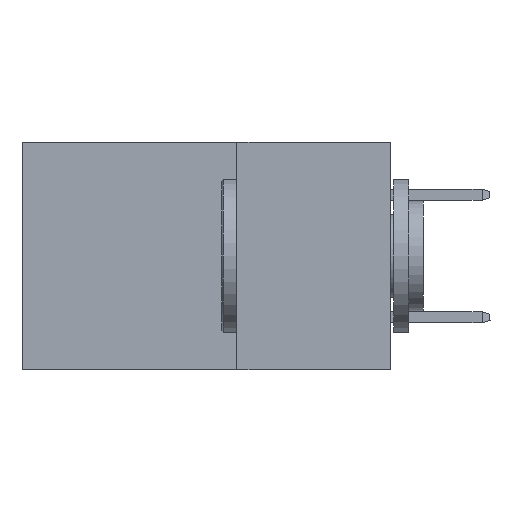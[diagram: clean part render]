
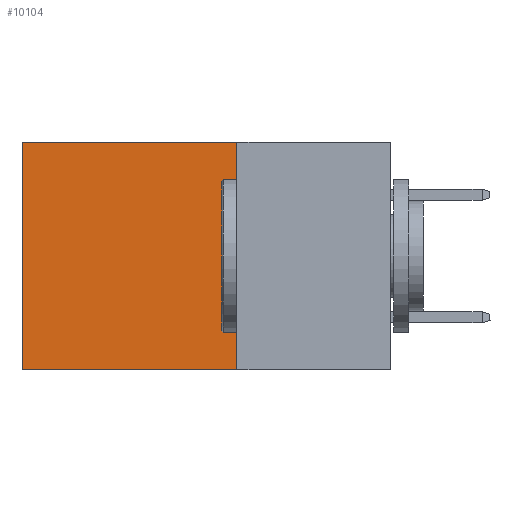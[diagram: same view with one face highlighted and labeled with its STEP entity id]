
A CAD part, left-side view. The second image highlights one B-rep face of the part: STEP entity #10104.
In plain terms, the highlighted planar face has unit normal (-1, 0, 0).
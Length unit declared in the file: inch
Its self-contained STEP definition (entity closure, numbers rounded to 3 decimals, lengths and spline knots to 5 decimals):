
#176 = LINE ( 'NONE', #5100, #5305 ) ;
#503 = AXIS2_PLACEMENT_3D ( 'NONE', #12562, #1805, #9003 ) ;
#543 = LINE ( 'NONE', #991, #11005 ) ;
#823 = LINE ( 'NONE', #1320, #3710 ) ;
#925 = DIRECTION ( 'NONE',  ( 0., 0., -1. ) ) ;
#991 = CARTESIAN_POINT ( 'NONE',  ( 0.2875, 0.25, 0. ) ) ;
#1142 = VERTEX_POINT ( 'NONE', #2001 ) ;
#1304 = DIRECTION ( 'NONE',  ( 0., 1., 0. ) ) ;
#1320 = CARTESIAN_POINT ( 'NONE',  ( 0.2875, 0.25, -0.37 ) ) ;
#1624 = LINE ( 'NONE', #2728, #6925 ) ;
#1805 = DIRECTION ( 'NONE',  ( 1., 0., 0. ) ) ;
#1990 = EDGE_CURVE ( 'NONE', #1142, #12833, #543, .T. ) ;
#2001 = CARTESIAN_POINT ( 'NONE',  ( 0.2875, 0.25, 0. ) ) ;
#2570 = ORIENTED_EDGE ( 'NONE', *, *, #1990, .F. ) ;
#2582 = EDGE_CURVE ( 'NONE', #1142, #4583, #176, .T. ) ;
#2728 = CARTESIAN_POINT ( 'NONE',  ( 0.2875, 0.6, 0. ) ) ;
#3677 = ORIENTED_EDGE ( 'NONE', *, *, #11192, .T. ) ;
#3710 = VECTOR ( 'NONE', #1304, 39.37008 ) ;
#3799 = DIRECTION ( 'NONE',  ( 0., 0., -1. ) ) ;
#4583 = VERTEX_POINT ( 'NONE', #12522 ) ;
#5075 = DIRECTION ( 'NONE',  ( 0., 1., 0. ) ) ;
#5100 = CARTESIAN_POINT ( 'NONE',  ( 0.2875, 0.25, 0. ) ) ;
#5305 = VECTOR ( 'NONE', #5075, 39.37008 ) ;
#5379 = CARTESIAN_POINT ( 'NONE',  ( 0.2875, 0.25, -0.37 ) ) ;
#6227 = EDGE_CURVE ( 'NONE', #12833, #11736, #823, .T. ) ;
#6925 = VECTOR ( 'NONE', #3799, 39.37008 ) ;
#7273 = FACE_OUTER_BOUND ( 'NONE', #10114, .T. ) ;
#8048 = PLANE ( 'NONE',  #503 ) ;
#9003 = DIRECTION ( 'NONE',  ( 0., 0., -1. ) ) ;
#9690 = CARTESIAN_POINT ( 'NONE',  ( 0.2875, 0.6, -0.37 ) ) ;
#10104 = ADVANCED_FACE ( 'NONE', ( #7273 ), #8048, .F. ) ;
#10114 = EDGE_LOOP ( 'NONE', ( #3677, #12733, #2570, #10648 ) ) ;
#10648 = ORIENTED_EDGE ( 'NONE', *, *, #2582, .T. ) ;
#11005 = VECTOR ( 'NONE', #925, 39.37008 ) ;
#11192 = EDGE_CURVE ( 'NONE', #4583, #11736, #1624, .T. ) ;
#11736 = VERTEX_POINT ( 'NONE', #9690 ) ;
#12522 = CARTESIAN_POINT ( 'NONE',  ( 0.2875, 0.6, 0. ) ) ;
#12562 = CARTESIAN_POINT ( 'NONE',  ( 0.2875, 0.25, 0. ) ) ;
#12733 = ORIENTED_EDGE ( 'NONE', *, *, #6227, .F. ) ;
#12833 = VERTEX_POINT ( 'NONE', #5379 ) ;
